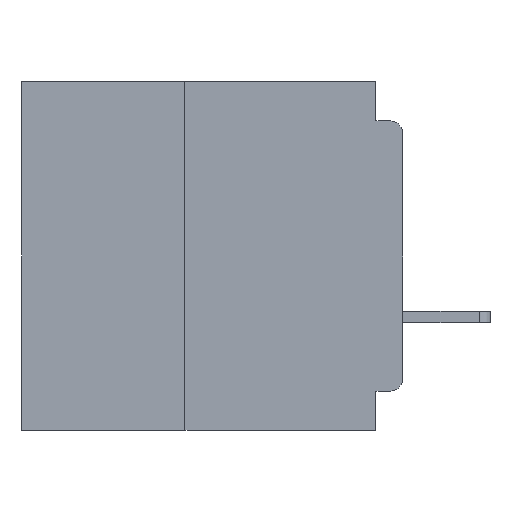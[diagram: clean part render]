
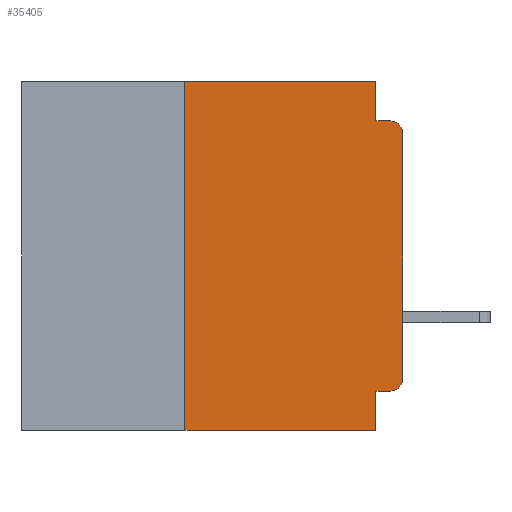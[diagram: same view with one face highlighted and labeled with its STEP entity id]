
A CAD part, left-side view. The second image highlights one B-rep face of the part: STEP entity #35405.
In plain terms, the highlighted planar face has unit normal (-1, 0, 0).
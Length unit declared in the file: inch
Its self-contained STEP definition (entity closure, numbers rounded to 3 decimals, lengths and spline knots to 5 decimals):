
#2575 = CARTESIAN_POINT ( 'NONE',  ( 0., 0.031, -0.4 ) ) ;
#2841 = VERTEX_POINT ( 'NONE', #8437 ) ;
#3250 = VERTEX_POINT ( 'NONE', #26169 ) ;
#3394 = VECTOR ( 'NONE', #40919, 39.37008 ) ;
#5008 = ORIENTED_EDGE ( 'NONE', *, *, #63837, .T. ) ;
#6099 = VECTOR ( 'NONE', #27888, 39.37008 ) ;
#7443 = ORIENTED_EDGE ( 'NONE', *, *, #27069, .F. ) ;
#8071 = EDGE_CURVE ( 'NONE', #48169, #38797, #50433, .T. ) ;
#8437 = CARTESIAN_POINT ( 'NONE',  ( 0., 0.015, -0.045 ) ) ;
#8967 = EDGE_LOOP ( 'NONE', ( #62109, #49900, #7443, #57946, #57735, #19055, #5008, #63358, #50424, #57262 ) ) ;
#9818 = DIRECTION ( 'NONE',  ( 0., 1., 0. ) ) ;
#10256 = CARTESIAN_POINT ( 'NONE',  ( 0., 0., -0.045 ) ) ;
#10904 = AXIS2_PLACEMENT_3D ( 'NONE', #46833, #15802, #52014 ) ;
#11587 = CARTESIAN_POINT ( 'NONE',  ( 0., 0.015, -0.355 ) ) ;
#13193 = PLANE ( 'NONE',  #55360 ) ;
#14841 = CARTESIAN_POINT ( 'NONE',  ( 0., 0.015, -0.34 ) ) ;
#15802 = DIRECTION ( 'NONE',  ( -1., 0., 0. ) ) ;
#17276 = DIRECTION ( 'NONE',  ( 0., 0., -1. ) ) ;
#17360 = CARTESIAN_POINT ( 'NONE',  ( 0., 0.031, -0.355 ) ) ;
#18766 = CARTESIAN_POINT ( 'NONE',  ( 0., 0., -0.34 ) ) ;
#19055 = ORIENTED_EDGE ( 'NONE', *, *, #8071, .F. ) ;
#20065 = DIRECTION ( 'NONE',  ( 0., 0., -1. ) ) ;
#21483 = VERTEX_POINT ( 'NONE', #54782 ) ;
#22166 = DIRECTION ( 'NONE',  ( 0., 0., 1. ) ) ;
#22669 = CARTESIAN_POINT ( 'NONE',  ( 0., 0.437, -0.4 ) ) ;
#22880 = LINE ( 'NONE', #29778, #52026 ) ;
#23670 = DIRECTION ( 'NONE',  ( 0., 0., -1. ) ) ;
#25951 = CIRCLE ( 'NONE', #57733, 0.015 ) ;
#25967 = CARTESIAN_POINT ( 'NONE',  ( 0., 0.031, -0.4 ) ) ;
#26169 = CARTESIAN_POINT ( 'NONE',  ( 0., 0.031, 0. ) ) ;
#26702 = CARTESIAN_POINT ( 'NONE',  ( 0., 0.25, -0.4 ) ) ;
#27069 = EDGE_CURVE ( 'NONE', #21483, #2841, #33613, .T. ) ;
#27096 = EDGE_CURVE ( 'NONE', #42454, #57249, #61087, .T. ) ;
#27888 = DIRECTION ( 'NONE',  ( 0., -1., 0. ) ) ;
#28247 = VERTEX_POINT ( 'NONE', #36491 ) ;
#28410 = EDGE_CURVE ( 'NONE', #38797, #3250, #34339, .T. ) ;
#28926 = EDGE_CURVE ( 'NONE', #59128, #28247, #22880, .T. ) ;
#29464 = LINE ( 'NONE', #48308, #56950 ) ;
#29778 = CARTESIAN_POINT ( 'NONE',  ( 0., 0., 0. ) ) ;
#30190 = EDGE_CURVE ( 'NONE', #39387, #59128, #25951, .T. ) ;
#30960 = DIRECTION ( 'NONE',  ( 0., -1., 0. ) ) ;
#31260 = EDGE_CURVE ( 'NONE', #28247, #2841, #38776, .T. ) ;
#33365 = VECTOR ( 'NONE', #9818, 39.37008 ) ;
#33613 = LINE ( 'NONE', #10256, #48991 ) ;
#34339 = LINE ( 'NONE', #51080, #3394 ) ;
#35405 = ADVANCED_FACE ( 'NONE', ( #45364 ), #13193, .F. ) ;
#36491 = CARTESIAN_POINT ( 'NONE',  ( 0., 0., -0.06 ) ) ;
#38776 = CIRCLE ( 'NONE', #10904, 0.015 ) ;
#38797 = VERTEX_POINT ( 'NONE', #42298 ) ;
#39387 = VERTEX_POINT ( 'NONE', #11587 ) ;
#40919 = DIRECTION ( 'NONE',  ( 0., -1., 0. ) ) ;
#42298 = CARTESIAN_POINT ( 'NONE',  ( 0., 0.25, 0. ) ) ;
#42454 = VERTEX_POINT ( 'NONE', #17360 ) ;
#45364 = FACE_OUTER_BOUND ( 'NONE', #8967, .T. ) ;
#46833 = CARTESIAN_POINT ( 'NONE',  ( 0., 0.015, -0.06 ) ) ;
#47540 = LINE ( 'NONE', #22669, #6099 ) ;
#48169 = VERTEX_POINT ( 'NONE', #26702 ) ;
#48308 = CARTESIAN_POINT ( 'NONE',  ( 0., 0.031, 0. ) ) ;
#48991 = VECTOR ( 'NONE', #30960, 39.37008 ) ;
#49494 = CARTESIAN_POINT ( 'NONE',  ( 0., 0.437, 0. ) ) ;
#49900 = ORIENTED_EDGE ( 'NONE', *, *, #31260, .T. ) ;
#50364 = LINE ( 'NONE', #66422, #33365 ) ;
#50424 = ORIENTED_EDGE ( 'NONE', *, *, #51875, .F. ) ;
#50433 = LINE ( 'NONE', #63530, #64122 ) ;
#50889 = EDGE_CURVE ( 'NONE', #3250, #21483, #29464, .T. ) ;
#51080 = CARTESIAN_POINT ( 'NONE',  ( 0., 0.437, 0. ) ) ;
#51088 = DIRECTION ( 'NONE',  ( -1., 0., 0. ) ) ;
#51875 = EDGE_CURVE ( 'NONE', #39387, #42454, #50364, .T. ) ;
#52014 = DIRECTION ( 'NONE',  ( 0., 0., -1. ) ) ;
#52026 = VECTOR ( 'NONE', #65873, 39.37008 ) ;
#54632 = DIRECTION ( 'NONE',  ( 1., 0., 0. ) ) ;
#54782 = CARTESIAN_POINT ( 'NONE',  ( 0., 0.031, -0.045 ) ) ;
#55360 = AXIS2_PLACEMENT_3D ( 'NONE', #49494, #54632, #23670 ) ;
#56950 = VECTOR ( 'NONE', #17276, 39.37008 ) ;
#57249 = VERTEX_POINT ( 'NONE', #2575 ) ;
#57262 = ORIENTED_EDGE ( 'NONE', *, *, #30190, .T. ) ;
#57733 = AXIS2_PLACEMENT_3D ( 'NONE', #14841, #51088, #20065 ) ;
#57735 = ORIENTED_EDGE ( 'NONE', *, *, #28410, .F. ) ;
#57946 = ORIENTED_EDGE ( 'NONE', *, *, #50889, .F. ) ;
#59128 = VERTEX_POINT ( 'NONE', #18766 ) ;
#59469 = VECTOR ( 'NONE', #62119, 39.37008 ) ;
#61087 = LINE ( 'NONE', #25967, #59469 ) ;
#62109 = ORIENTED_EDGE ( 'NONE', *, *, #28926, .T. ) ;
#62119 = DIRECTION ( 'NONE',  ( 0., 0., -1. ) ) ;
#63358 = ORIENTED_EDGE ( 'NONE', *, *, #27096, .F. ) ;
#63530 = CARTESIAN_POINT ( 'NONE',  ( 0., 0.25, -0.4 ) ) ;
#63837 = EDGE_CURVE ( 'NONE', #48169, #57249, #47540, .T. ) ;
#64122 = VECTOR ( 'NONE', #22166, 39.37008 ) ;
#65873 = DIRECTION ( 'NONE',  ( 0., 0., 1. ) ) ;
#66422 = CARTESIAN_POINT ( 'NONE',  ( 0., 0., -0.355 ) ) ;
